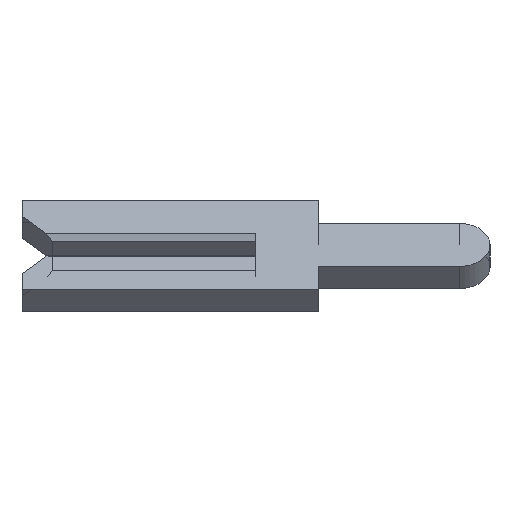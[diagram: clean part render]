
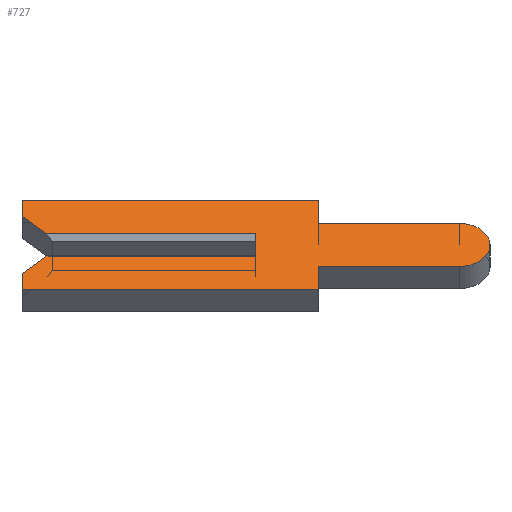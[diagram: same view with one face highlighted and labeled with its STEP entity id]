
A CAD part, left-side view. The second image highlights one B-rep face of the part: STEP entity #727.
In plain terms, the highlighted face is planar.
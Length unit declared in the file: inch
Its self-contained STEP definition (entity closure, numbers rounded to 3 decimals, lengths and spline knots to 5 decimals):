
#2 = EDGE_CURVE ( 'NONE', #1154, #857, #562, .T. ) ;
#72 = VERTEX_POINT ( 'NONE', #570 ) ;
#76 = DIRECTION ( 'NONE',  ( 0., 0., -1. ) ) ;
#102 = CIRCLE ( 'NONE', #573, 0.0195 ) ;
#111 = EDGE_CURVE ( 'NONE', #2701, #491, #1163, .T. ) ;
#119 = CARTESIAN_POINT ( 'NONE',  ( -0.01, -0.04, 0.04 ) ) ;
#151 = ORIENTED_EDGE ( 'NONE', *, *, #736, .F. ) ;
#153 = CARTESIAN_POINT ( 'NONE',  ( -0.01, 0.134, 0.01 ) ) ;
#184 = DIRECTION ( 'NONE',  ( 0., 0., 1. ) ) ;
#186 = CARTESIAN_POINT ( 'NONE',  ( -0.01, 0.15, -0.04 ) ) ;
#214 = VECTOR ( 'NONE', #1620, 39.37008 ) ;
#253 = VECTOR ( 'NONE', #1208, 39.37008 ) ;
#272 = DIRECTION ( 'NONE',  ( 1., 0., 0. ) ) ;
#288 = LINE ( 'NONE', #2336, #2697 ) ;
#296 = EDGE_LOOP ( 'NONE', ( #451, #2585, #1283, #1908, #1679, #1973, #3031, #2876, #1985, #2503, #1249, #151, #2059, #2706 ) ) ;
#297 = CARTESIAN_POINT ( 'NONE',  ( -0.01, -0.04, -0.04 ) ) ;
#324 = VERTEX_POINT ( 'NONE', #153 ) ;
#380 = CARTESIAN_POINT ( 'NONE',  ( -0.01, 0.15, 0.026 ) ) ;
#402 = LINE ( 'NONE', #297, #2731 ) ;
#443 = VECTOR ( 'NONE', #1348, 39.37008 ) ;
#448 = CARTESIAN_POINT ( 'NONE',  ( -0.01, 0.15, 0.01 ) ) ;
#451 = ORIENTED_EDGE ( 'NONE', *, *, #977, .T. ) ;
#491 = VERTEX_POINT ( 'NONE', #2039 ) ;
#557 = CARTESIAN_POINT ( 'NONE',  ( -0.01, -0.04, -0.04 ) ) ;
#562 = LINE ( 'NONE', #1524, #2431 ) ;
#570 = CARTESIAN_POINT ( 'NONE',  ( -0.01, 0.15, -0.04 ) ) ;
#573 = AXIS2_PLACEMENT_3D ( 'NONE', #2873, #272, #1682 ) ;
#596 = EDGE_CURVE ( 'NONE', #1049, #72, #932, .T. ) ;
#599 = VECTOR ( 'NONE', #1297, 39.37008 ) ;
#610 = CARTESIAN_POINT ( 'NONE',  ( -0.01, -0.04, -0.0195 ) ) ;
#676 = EDGE_CURVE ( 'NONE', #324, #2810, #288, .T. ) ;
#679 = VERTEX_POINT ( 'NONE', #885 ) ;
#727 = ADVANCED_FACE ( 'NONE', ( #1869 ), #1407, .F. ) ;
#736 = EDGE_CURVE ( 'NONE', #1402, #1154, #2427, .T. ) ;
#828 = AXIS2_PLACEMENT_3D ( 'NONE', #2581, #1885, #1876 ) ;
#857 = VERTEX_POINT ( 'NONE', #1148 ) ;
#885 = CARTESIAN_POINT ( 'NONE',  ( -0.01, -0.1305, 0.0195 ) ) ;
#887 = VECTOR ( 'NONE', #2857, 39.37008 ) ;
#932 = LINE ( 'NONE', #186, #214 ) ;
#946 = CARTESIAN_POINT ( 'NONE',  ( -0.01, -0.1305, -0.01 ) ) ;
#977 = EDGE_CURVE ( 'NONE', #324, #491, #2574, .T. ) ;
#1049 = VERTEX_POINT ( 'NONE', #557 ) ;
#1054 = CARTESIAN_POINT ( 'NONE',  ( -0.01, 0., 0.0065 ) ) ;
#1081 = CARTESIAN_POINT ( 'NONE',  ( -0.01, 0.1305, -0.0065 ) ) ;
#1140 = EDGE_CURVE ( 'NONE', #2128, #2576, #2771, .T. ) ;
#1148 = CARTESIAN_POINT ( 'NONE',  ( -0.01, -0.04, 0.0195 ) ) ;
#1154 = VERTEX_POINT ( 'NONE', #119 ) ;
#1163 = LINE ( 'NONE', #1054, #599 ) ;
#1183 = EDGE_CURVE ( 'NONE', #2854, #2779, #1277, .T. ) ;
#1208 = DIRECTION ( 'NONE',  ( 0., -1., 0. ) ) ;
#1249 = ORIENTED_EDGE ( 'NONE', *, *, #2, .F. ) ;
#1250 = EDGE_CURVE ( 'NONE', #2810, #1402, #1544, .T. ) ;
#1277 = LINE ( 'NONE', #1081, #443 ) ;
#1283 = ORIENTED_EDGE ( 'NONE', *, *, #2152, .F. ) ;
#1297 = DIRECTION ( 'NONE',  ( 0., 0., 1. ) ) ;
#1308 = DIRECTION ( 'NONE',  ( 0., 1., 0. ) ) ;
#1348 = DIRECTION ( 'NONE',  ( 0., -0.707, 0.707 ) ) ;
#1353 = VECTOR ( 'NONE', #1844, 39.37008 ) ;
#1402 = VERTEX_POINT ( 'NONE', #2580 ) ;
#1407 = PLANE ( 'NONE',  #828 ) ;
#1472 = EDGE_CURVE ( 'NONE', #857, #679, #2850, .T. ) ;
#1490 = CARTESIAN_POINT ( 'NONE',  ( -0.01, -0.1305, -0.0195 ) ) ;
#1502 = CARTESIAN_POINT ( 'NONE',  ( -0.01, 0., -0.01 ) ) ;
#1524 = CARTESIAN_POINT ( 'NONE',  ( -0.01, -0.04, 0.04 ) ) ;
#1538 = DIRECTION ( 'NONE',  ( 0., 0., -1. ) ) ;
#1544 = LINE ( 'NONE', #380, #1353 ) ;
#1620 = DIRECTION ( 'NONE',  ( 0., 1., 0. ) ) ;
#1624 = EDGE_CURVE ( 'NONE', #72, #2854, #1688, .T. ) ;
#1679 = ORIENTED_EDGE ( 'NONE', *, *, #1624, .F. ) ;
#1682 = DIRECTION ( 'NONE',  ( 0., 0., -1. ) ) ;
#1688 = LINE ( 'NONE', #2610, #1938 ) ;
#1752 = CARTESIAN_POINT ( 'NONE',  ( -0.01, 0.134, -0.01 ) ) ;
#1844 = DIRECTION ( 'NONE',  ( 0., 0., 1. ) ) ;
#1853 = DIRECTION ( 'NONE',  ( 0., 0.707, 0.707 ) ) ;
#1869 = FACE_OUTER_BOUND ( 'NONE', #296, .T. ) ;
#1876 = DIRECTION ( 'NONE',  ( 0., 0., -1. ) ) ;
#1885 = DIRECTION ( 'NONE',  ( 1., 0., 0. ) ) ;
#1908 = ORIENTED_EDGE ( 'NONE', *, *, #1183, .F. ) ;
#1938 = VECTOR ( 'NONE', #184, 39.37008 ) ;
#1973 = ORIENTED_EDGE ( 'NONE', *, *, #596, .F. ) ;
#1984 = CARTESIAN_POINT ( 'NONE',  ( -0.01, 0.15, -0.026 ) ) ;
#1985 = ORIENTED_EDGE ( 'NONE', *, *, #2017, .F. ) ;
#2017 = EDGE_CURVE ( 'NONE', #679, #2128, #102, .T. ) ;
#2039 = CARTESIAN_POINT ( 'NONE',  ( -0.01, 0., 0.01 ) ) ;
#2056 = VECTOR ( 'NONE', #2377, 39.37008 ) ;
#2059 = ORIENTED_EDGE ( 'NONE', *, *, #1250, .F. ) ;
#2123 = LINE ( 'NONE', #946, #2804 ) ;
#2125 = VECTOR ( 'NONE', #1308, 39.37008 ) ;
#2128 = VERTEX_POINT ( 'NONE', #1490 ) ;
#2152 = EDGE_CURVE ( 'NONE', #2779, #2701, #2123, .T. ) ;
#2163 = DIRECTION ( 'NONE',  ( 0., -1., 0. ) ) ;
#2336 = CARTESIAN_POINT ( 'NONE',  ( -0.01, 0.1305, 0.0065 ) ) ;
#2377 = DIRECTION ( 'NONE',  ( 0., -1., 0. ) ) ;
#2427 = LINE ( 'NONE', #2811, #2056 ) ;
#2431 = VECTOR ( 'NONE', #76, 39.37008 ) ;
#2452 = CARTESIAN_POINT ( 'NONE',  ( -0.01, -0.04, -0.0195 ) ) ;
#2494 = EDGE_CURVE ( 'NONE', #2576, #1049, #402, .T. ) ;
#2503 = ORIENTED_EDGE ( 'NONE', *, *, #1472, .F. ) ;
#2574 = LINE ( 'NONE', #448, #253 ) ;
#2576 = VERTEX_POINT ( 'NONE', #2452 ) ;
#2580 = CARTESIAN_POINT ( 'NONE',  ( -0.01, 0.15, 0.04 ) ) ;
#2581 = CARTESIAN_POINT ( 'NONE',  ( -0.01, -0.1305, 0. ) ) ;
#2585 = ORIENTED_EDGE ( 'NONE', *, *, #111, .F. ) ;
#2610 = CARTESIAN_POINT ( 'NONE',  ( -0.01, 0.15, -0.026 ) ) ;
#2697 = VECTOR ( 'NONE', #1853, 39.37008 ) ;
#2701 = VERTEX_POINT ( 'NONE', #1502 ) ;
#2706 = ORIENTED_EDGE ( 'NONE', *, *, #676, .F. ) ;
#2731 = VECTOR ( 'NONE', #1538, 39.37008 ) ;
#2771 = LINE ( 'NONE', #610, #2125 ) ;
#2779 = VERTEX_POINT ( 'NONE', #1752 ) ;
#2804 = VECTOR ( 'NONE', #2163, 39.37008 ) ;
#2810 = VERTEX_POINT ( 'NONE', #2962 ) ;
#2811 = CARTESIAN_POINT ( 'NONE',  ( -0.01, 0.15, 0.04 ) ) ;
#2830 = CARTESIAN_POINT ( 'NONE',  ( -0.01, -0.04, 0.0195 ) ) ;
#2850 = LINE ( 'NONE', #2830, #887 ) ;
#2854 = VERTEX_POINT ( 'NONE', #1984 ) ;
#2857 = DIRECTION ( 'NONE',  ( 0., -1., 0. ) ) ;
#2873 = CARTESIAN_POINT ( 'NONE',  ( -0.01, -0.1305, 0. ) ) ;
#2876 = ORIENTED_EDGE ( 'NONE', *, *, #1140, .F. ) ;
#2962 = CARTESIAN_POINT ( 'NONE',  ( -0.01, 0.15, 0.026 ) ) ;
#3031 = ORIENTED_EDGE ( 'NONE', *, *, #2494, .F. ) ;
